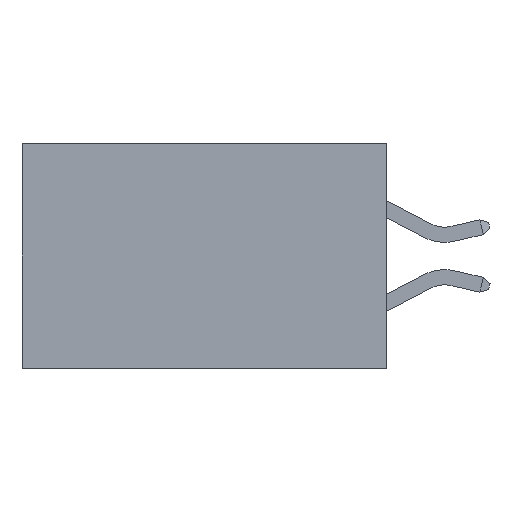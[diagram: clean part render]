
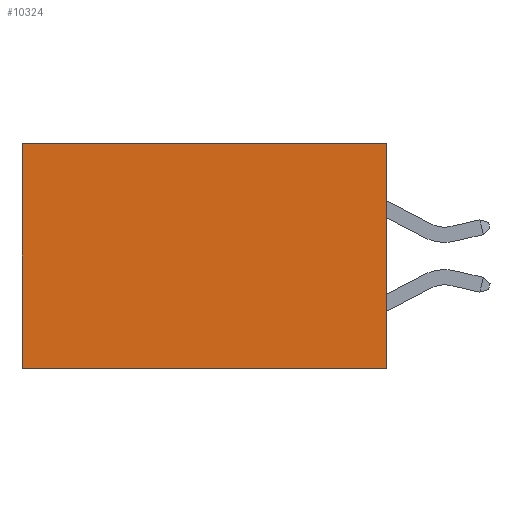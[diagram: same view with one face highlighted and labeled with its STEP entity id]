
A CAD part, left-side view. The second image highlights one B-rep face of the part: STEP entity #10324.
In plain terms, the highlighted planar face has unit normal (-1, 0, 0).
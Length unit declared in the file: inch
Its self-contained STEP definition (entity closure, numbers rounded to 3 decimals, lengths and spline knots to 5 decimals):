
#1028 = ORIENTED_EDGE ( 'NONE', *, *, #4449, .T. ) ;
#1043 = CARTESIAN_POINT ( 'NONE',  ( 0.298, 0., 0. ) ) ;
#1189 = DIRECTION ( 'NONE',  ( 0., 0., -1. ) ) ;
#1349 = DIRECTION ( 'NONE',  ( 0., 0., -1. ) ) ;
#1860 = EDGE_CURVE ( 'NONE', #1918, #7110, #6660, .T. ) ;
#1918 = VERTEX_POINT ( 'NONE', #6736 ) ;
#2077 = ORIENTED_EDGE ( 'NONE', *, *, #9374, .F. ) ;
#2149 = DIRECTION ( 'NONE',  ( 0., 0., -1. ) ) ;
#2397 = CARTESIAN_POINT ( 'NONE',  ( 0.298, 0., 0. ) ) ;
#3329 = CARTESIAN_POINT ( 'NONE',  ( 0.298, 0., -0.37 ) ) ;
#3982 = CARTESIAN_POINT ( 'NONE',  ( 0.298, 0., 0. ) ) ;
#4050 = VECTOR ( 'NONE', #1189, 39.37008 ) ;
#4449 = EDGE_CURVE ( 'NONE', #7110, #7318, #7996, .T. ) ;
#4791 = CARTESIAN_POINT ( 'NONE',  ( 0.298, 0.6, -0.37 ) ) ;
#6150 = VECTOR ( 'NONE', #2149, 39.37008 ) ;
#6565 = DIRECTION ( 'NONE',  ( 1., 0., 0. ) ) ;
#6660 = LINE ( 'NONE', #2397, #8572 ) ;
#6736 = CARTESIAN_POINT ( 'NONE',  ( 0.298, 0., 0. ) ) ;
#6811 = DIRECTION ( 'NONE',  ( 0., 1., 0. ) ) ;
#7110 = VERTEX_POINT ( 'NONE', #8402 ) ;
#7281 = EDGE_CURVE ( 'NONE', #1918, #9791, #9148, .T. ) ;
#7318 = VERTEX_POINT ( 'NONE', #4791 ) ;
#7901 = VECTOR ( 'NONE', #9473, 39.37008 ) ;
#7996 = LINE ( 'NONE', #10616, #4050 ) ;
#8402 = CARTESIAN_POINT ( 'NONE',  ( 0.298, 0.6, 0. ) ) ;
#8572 = VECTOR ( 'NONE', #6811, 39.37008 ) ;
#8613 = FACE_OUTER_BOUND ( 'NONE', #10760, .T. ) ;
#9148 = LINE ( 'NONE', #1043, #6150 ) ;
#9374 = EDGE_CURVE ( 'NONE', #9791, #7318, #10193, .T. ) ;
#9473 = DIRECTION ( 'NONE',  ( 0., 1., 0. ) ) ;
#9648 = AXIS2_PLACEMENT_3D ( 'NONE', #3982, #6565, #1349 ) ;
#9791 = VERTEX_POINT ( 'NONE', #9936 ) ;
#9936 = CARTESIAN_POINT ( 'NONE',  ( 0.298, 0., -0.37 ) ) ;
#10193 = LINE ( 'NONE', #3329, #7901 ) ;
#10324 = ADVANCED_FACE ( 'NONE', ( #8613 ), #10857, .F. ) ;
#10616 = CARTESIAN_POINT ( 'NONE',  ( 0.298, 0.6, 0. ) ) ;
#10671 = ORIENTED_EDGE ( 'NONE', *, *, #1860, .T. ) ;
#10686 = ORIENTED_EDGE ( 'NONE', *, *, #7281, .F. ) ;
#10760 = EDGE_LOOP ( 'NONE', ( #1028, #2077, #10686, #10671 ) ) ;
#10857 = PLANE ( 'NONE',  #9648 ) ;
